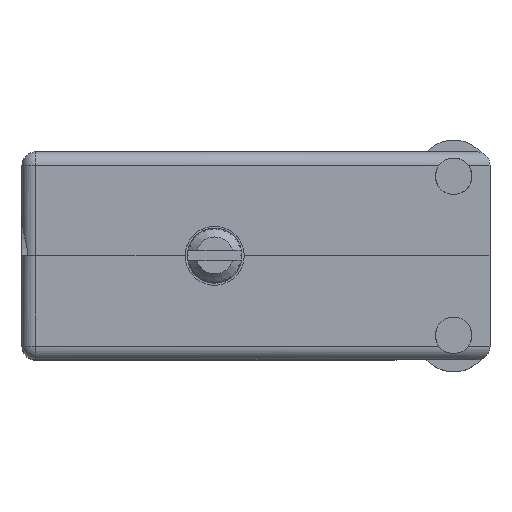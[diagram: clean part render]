
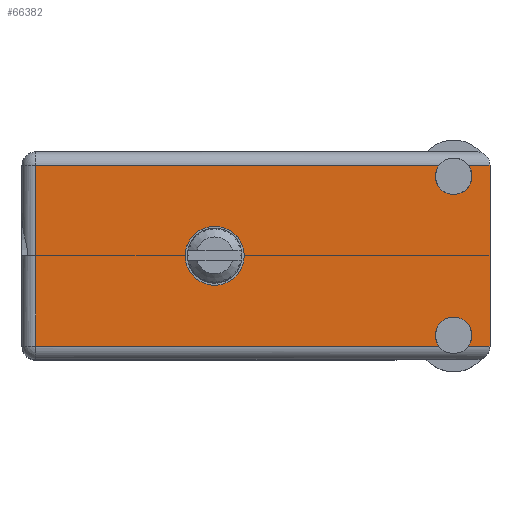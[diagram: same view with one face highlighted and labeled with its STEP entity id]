
A CAD part, top view. The second image highlights one B-rep face of the part: STEP entity #66382.
In plain terms, the highlighted face is planar.
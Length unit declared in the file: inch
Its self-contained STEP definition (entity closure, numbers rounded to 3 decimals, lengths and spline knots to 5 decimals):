
#2146 = CARTESIAN_POINT ( 'NONE',  ( 0., 0.806, 0. ) ) ;
#2603 = VECTOR ( 'NONE', #17751, 39.37008 ) ;
#3382 = EDGE_LOOP ( 'NONE', ( #40371, #117091, #161561, #196012, #77471, #58496, #20488, #196246, #113252, #73307 ) ) ;
#4552 = DIRECTION ( 'NONE',  ( 0., 1., 0. ) ) ;
#8059 = DIRECTION ( 'NONE',  ( 0., 0., 1. ) ) ;
#9591 = VERTEX_POINT ( 'NONE', #99478 ) ;
#12044 = CARTESIAN_POINT ( 'NONE',  ( 0.9465, 0.806, 0.3575 ) ) ;
#12789 = EDGE_CURVE ( 'NONE', #31753, #9591, #162158, .T. ) ;
#13306 = EDGE_CURVE ( 'NONE', #111486, #82113, #176452, .T. ) ;
#17741 = CARTESIAN_POINT ( 'NONE',  ( 0.9465, 0.806, 0.3105 ) ) ;
#17751 = DIRECTION ( 'NONE',  ( -1., 0., 0. ) ) ;
#20488 = ORIENTED_EDGE ( 'NONE', *, *, #12789, .F. ) ;
#21020 = FACE_OUTER_BOUND ( 'NONE', #3382, .T. ) ;
#23374 = CARTESIAN_POINT ( 'NONE',  ( 0.87187, 0.806, 0.3105 ) ) ;
#23963 = EDGE_CURVE ( 'NONE', #62636, #26955, #35768, .T. ) ;
#26955 = VERTEX_POINT ( 'NONE', #127510 ) ;
#27353 = CARTESIAN_POINT ( 'NONE',  ( 0.8215, 0.806, 0.2735 ) ) ;
#29513 = LINE ( 'NONE', #17741, #147633 ) ;
#31753 = VERTEX_POINT ( 'NONE', #134746 ) ;
#34916 = EDGE_CURVE ( 'NONE', #43283, #175560, #29513, .T. ) ;
#35768 = LINE ( 'NONE', #99449, #50309 ) ;
#38729 = EDGE_CURVE ( 'NONE', #181712, #26955, #108704, .T. ) ;
#40371 = ORIENTED_EDGE ( 'NONE', *, *, #34916, .T. ) ;
#43283 = VERTEX_POINT ( 'NONE', #113989 ) ;
#43464 = VERTEX_POINT ( 'NONE', #117813 ) ;
#43542 = DIRECTION ( 'NONE',  ( 0., 0., 1. ) ) ;
#45108 = DIRECTION ( 'NONE',  ( 0., 0., 1. ) ) ;
#47978 = EDGE_CURVE ( 'NONE', #68056, #43464, #114515, .T. ) ;
#50309 = VECTOR ( 'NONE', #116187, 39.37008 ) ;
#51396 = DIRECTION ( 'NONE',  ( 0., 0., 1. ) ) ;
#53433 = EDGE_CURVE ( 'NONE', #43464, #68056, #144918, .T. ) ;
#57510 = VECTOR ( 'NONE', #8059, 39.37008 ) ;
#58496 = ORIENTED_EDGE ( 'NONE', *, *, #178168, .T. ) ;
#61413 = DIRECTION ( 'NONE',  ( 0., 1., 0. ) ) ;
#62374 = VERTEX_POINT ( 'NONE', #124547 ) ;
#62636 = VERTEX_POINT ( 'NONE', #23374 ) ;
#65453 = DIRECTION ( 'NONE',  ( 0., 0., 1. ) ) ;
#66382 = ADVANCED_FACE ( 'NONE', ( #144023, #21020 ), #171910, .T. ) ;
#68056 = VERTEX_POINT ( 'NONE', #138048 ) ;
#68919 = CARTESIAN_POINT ( 'NONE',  ( 0., 0.806, 0. ) ) ;
#71600 = EDGE_CURVE ( 'NONE', #111486, #31753, #129804, .T. ) ;
#72742 = DIRECTION ( 'NONE',  ( 0., 0., 1. ) ) ;
#73307 = ORIENTED_EDGE ( 'NONE', *, *, #96734, .T. ) ;
#77471 = ORIENTED_EDGE ( 'NONE', *, *, #38729, .F. ) ;
#82113 = VERTEX_POINT ( 'NONE', #131634 ) ;
#89715 = DIRECTION ( 'NONE',  ( 0., 1., 0. ) ) ;
#93772 = AXIS2_PLACEMENT_3D ( 'NONE', #186089, #61413, #109266 ) ;
#96734 = EDGE_CURVE ( 'NONE', #82113, #43283, #197357, .T. ) ;
#96795 = AXIS2_PLACEMENT_3D ( 'NONE', #121994, #89715, #45108 ) ;
#97777 = CARTESIAN_POINT ( 'NONE',  ( -0.6155, 0.806, -0.3575 ) ) ;
#99449 = CARTESIAN_POINT ( 'NONE',  ( 0.9465, 0.806, 0.3105 ) ) ;
#99478 = CARTESIAN_POINT ( 'NONE',  ( 0.87187, 0.806, -0.3105 ) ) ;
#102976 = EDGE_CURVE ( 'NONE', #62636, #62374, #155452, .T. ) ;
#108704 = LINE ( 'NONE', #12044, #161664 ) ;
#109266 = DIRECTION ( 'NONE',  ( -1., 0., 0. ) ) ;
#111486 = VERTEX_POINT ( 'NONE', #130733 ) ;
#112367 = DIRECTION ( 'NONE',  ( 0., 0., 1. ) ) ;
#113027 = AXIS2_PLACEMENT_3D ( 'NONE', #68919, #143753, #51396 ) ;
#113252 = ORIENTED_EDGE ( 'NONE', *, *, #13306, .T. ) ;
#113989 = CARTESIAN_POINT ( 'NONE',  ( -0.6155, 0.806, 0.3105 ) ) ;
#114515 = CIRCLE ( 'NONE', #140598, 0.1015 ) ;
#116187 = DIRECTION ( 'NONE',  ( 1., 0., 0. ) ) ;
#117091 = ORIENTED_EDGE ( 'NONE', *, *, #123709, .F. ) ;
#117813 = CARTESIAN_POINT ( 'NONE',  ( 0., 0.806, 0.1015 ) ) ;
#121994 = CARTESIAN_POINT ( 'NONE',  ( 0.8215, 0.806, -0.2735 ) ) ;
#123094 = CARTESIAN_POINT ( 'NONE',  ( -0.6625, 0.806, -0.3105 ) ) ;
#123709 = EDGE_CURVE ( 'NONE', #62374, #175560, #145747, .T. ) ;
#124547 = CARTESIAN_POINT ( 'NONE',  ( 0.8215, 0.806, 0.211 ) ) ;
#124885 = CARTESIAN_POINT ( 'NONE',  ( -0.6625, 0.806, -0.3105 ) ) ;
#127123 = DIRECTION ( 'NONE',  ( 0., 0., 1. ) ) ;
#127510 = CARTESIAN_POINT ( 'NONE',  ( 0.9465, 0.806, 0.3105 ) ) ;
#129804 = CIRCLE ( 'NONE', #194116, 0.0625 ) ;
#130733 = CARTESIAN_POINT ( 'NONE',  ( 0.77113, 0.806, -0.3105 ) ) ;
#131634 = CARTESIAN_POINT ( 'NONE',  ( -0.6155, 0.806, -0.3105 ) ) ;
#134746 = CARTESIAN_POINT ( 'NONE',  ( 0.8215, 0.806, -0.211 ) ) ;
#137842 = AXIS2_PLACEMENT_3D ( 'NONE', #27353, #168850, #43542 ) ;
#138048 = CARTESIAN_POINT ( 'NONE',  ( 0., 0.806, -0.1015 ) ) ;
#138605 = DIRECTION ( 'NONE',  ( -1., 0., 0. ) ) ;
#140598 = AXIS2_PLACEMENT_3D ( 'NONE', #2146, #157785, #65453 ) ;
#143753 = DIRECTION ( 'NONE',  ( 0., 1., 0. ) ) ;
#144023 = FACE_BOUND ( 'NONE', #162925, .T. ) ;
#144918 = CIRCLE ( 'NONE', #113027, 0.1015 ) ;
#145130 = VECTOR ( 'NONE', #138605, 39.37008 ) ;
#145747 = CIRCLE ( 'NONE', #137842, 0.0625 ) ;
#147633 = VECTOR ( 'NONE', #188224, 39.37008 ) ;
#152110 = LINE ( 'NONE', #124885, #2603 ) ;
#155452 = CIRCLE ( 'NONE', #161938, 0.0625 ) ;
#156142 = CARTESIAN_POINT ( 'NONE',  ( 0.8215, 0.806, -0.2735 ) ) ;
#157785 = DIRECTION ( 'NONE',  ( 0., 1., 0. ) ) ;
#161561 = ORIENTED_EDGE ( 'NONE', *, *, #102976, .F. ) ;
#161664 = VECTOR ( 'NONE', #72742, 39.37008 ) ;
#161938 = AXIS2_PLACEMENT_3D ( 'NONE', #187902, #4552, #112367 ) ;
#162158 = CIRCLE ( 'NONE', #96795, 0.0625 ) ;
#162925 = EDGE_LOOP ( 'NONE', ( #168931, #197546 ) ) ;
#168850 = DIRECTION ( 'NONE',  ( 0., 1., 0. ) ) ;
#168931 = ORIENTED_EDGE ( 'NONE', *, *, #53433, .F. ) ;
#169935 = CARTESIAN_POINT ( 'NONE',  ( 0.77113, 0.806, 0.3105 ) ) ;
#171910 = PLANE ( 'NONE',  #93772 ) ;
#174226 = DIRECTION ( 'NONE',  ( 0., 1., 0. ) ) ;
#175560 = VERTEX_POINT ( 'NONE', #169935 ) ;
#176452 = LINE ( 'NONE', #123094, #145130 ) ;
#178168 = EDGE_CURVE ( 'NONE', #181712, #9591, #152110, .T. ) ;
#181712 = VERTEX_POINT ( 'NONE', #198987 ) ;
#186089 = CARTESIAN_POINT ( 'NONE',  ( -0.6625, 0.806, -0.3575 ) ) ;
#187902 = CARTESIAN_POINT ( 'NONE',  ( 0.8215, 0.806, 0.2735 ) ) ;
#188224 = DIRECTION ( 'NONE',  ( 1., 0., 0. ) ) ;
#194116 = AXIS2_PLACEMENT_3D ( 'NONE', #156142, #174226, #127123 ) ;
#196012 = ORIENTED_EDGE ( 'NONE', *, *, #23963, .T. ) ;
#196246 = ORIENTED_EDGE ( 'NONE', *, *, #71600, .F. ) ;
#197357 = LINE ( 'NONE', #97777, #57510 ) ;
#197546 = ORIENTED_EDGE ( 'NONE', *, *, #47978, .F. ) ;
#198987 = CARTESIAN_POINT ( 'NONE',  ( 0.9465, 0.806, -0.3105 ) ) ;
